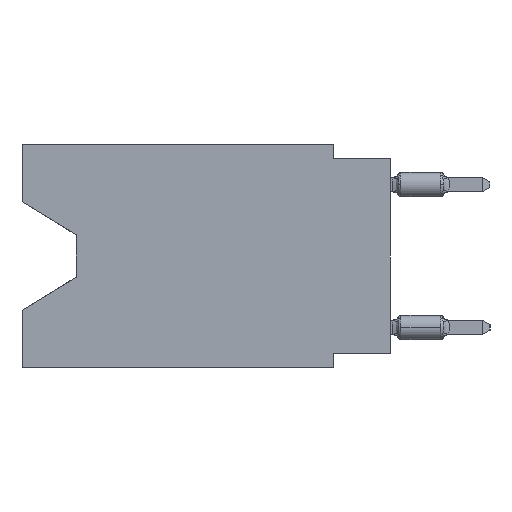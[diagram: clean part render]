
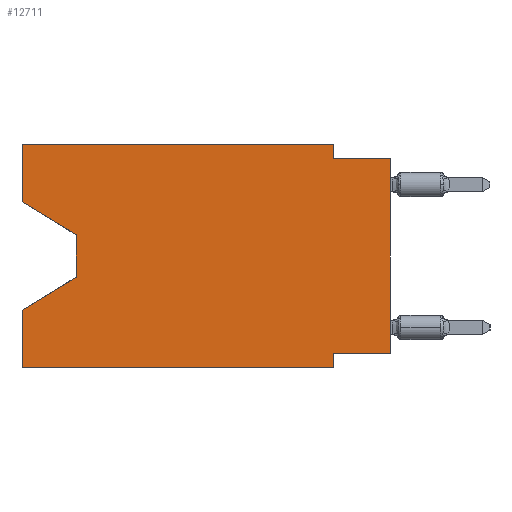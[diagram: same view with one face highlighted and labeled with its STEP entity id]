
A CAD part, left-side view. The second image highlights one B-rep face of the part: STEP entity #12711.
In plain terms, the highlighted planar face has unit normal (-1, 0, 0).
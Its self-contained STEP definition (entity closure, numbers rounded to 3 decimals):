
#188 = CARTESIAN_POINT ( 'NONE',  ( 0., 16.383, 0. ) ) ;
#466 = DIRECTION ( 'NONE',  ( 0., 0., -1. ) ) ;
#687 = EDGE_CURVE ( 'NONE', #22257, #24247, #35026, .T. ) ;
#1067 = CARTESIAN_POINT ( 'NONE',  ( 0., 2.54, -9.271 ) ) ;
#1289 = ORIENTED_EDGE ( 'NONE', *, *, #43319, .F. ) ;
#1474 = CARTESIAN_POINT ( 'NONE',  ( 0., 0., -9.271 ) ) ;
#1740 = CARTESIAN_POINT ( 'NONE',  ( 0., 2.54, 0. ) ) ;
#2173 = CARTESIAN_POINT ( 'NONE',  ( 0., 16.383, -2.546 ) ) ;
#2188 = ORIENTED_EDGE ( 'NONE', *, *, #28853, .F. ) ;
#2395 = DIRECTION ( 'NONE',  ( 0., -0.855, -0.519 ) ) ;
#2905 = DIRECTION ( 'NONE',  ( 0., 0., 1. ) ) ;
#3625 = LINE ( 'NONE', #37755, #48003 ) ;
#3892 = ORIENTED_EDGE ( 'NONE', *, *, #29347, .T. ) ;
#5490 = DIRECTION ( 'NONE',  ( 0., -1., 0. ) ) ;
#5667 = CARTESIAN_POINT ( 'NONE',  ( 0., 16.383, -9.906 ) ) ;
#5978 = AXIS2_PLACEMENT_3D ( 'NONE', #27079, #42142, #466 ) ;
#7020 = FACE_OUTER_BOUND ( 'NONE', #26149, .T. ) ;
#7174 = CARTESIAN_POINT ( 'NONE',  ( 0., 16.383, -2.546 ) ) ;
#7185 = CARTESIAN_POINT ( 'NONE',  ( 0., 16.383, 0. ) ) ;
#8102 = DIRECTION ( 'NONE',  ( 0., 0., -1. ) ) ;
#8670 = DIRECTION ( 'NONE',  ( 0., 0.855, -0.519 ) ) ;
#8674 = DIRECTION ( 'NONE',  ( 0., 0., 1. ) ) ;
#8768 = EDGE_CURVE ( 'NONE', #19900, #25504, #31499, .T. ) ;
#8898 = ORIENTED_EDGE ( 'NONE', *, *, #8768, .T. ) ;
#9522 = CARTESIAN_POINT ( 'NONE',  ( 0., 13.97, -4.013 ) ) ;
#9997 = LINE ( 'NONE', #21544, #36901 ) ;
#10736 = CARTESIAN_POINT ( 'NONE',  ( 0., 16.383, 0. ) ) ;
#11682 = CARTESIAN_POINT ( 'NONE',  ( 0., 0., -9.271 ) ) ;
#11773 = VECTOR ( 'NONE', #8674, 1000. ) ;
#12279 = VECTOR ( 'NONE', #8102, 1000. ) ;
#12711 = ADVANCED_FACE ( 'NONE', ( #7020 ), #19061, .F. ) ;
#13603 = VECTOR ( 'NONE', #16698, 1000. ) ;
#13773 = DIRECTION ( 'NONE',  ( 0., 1., 0. ) ) ;
#15073 = ORIENTED_EDGE ( 'NONE', *, *, #20942, .F. ) ;
#15950 = CARTESIAN_POINT ( 'NONE',  ( 0., 0., 0. ) ) ;
#16143 = EDGE_CURVE ( 'NONE', #34106, #33599, #21721, .T. ) ;
#16698 = DIRECTION ( 'NONE',  ( 0., -1., 0. ) ) ;
#16947 = EDGE_CURVE ( 'NONE', #25840, #47606, #9997, .T. ) ;
#17145 = ORIENTED_EDGE ( 'NONE', *, *, #46094, .F. ) ;
#18259 = VECTOR ( 'NONE', #26549, 1000. ) ;
#18798 = ORIENTED_EDGE ( 'NONE', *, *, #22177, .F. ) ;
#19061 = PLANE ( 'NONE',  #5978 ) ;
#19886 = CARTESIAN_POINT ( 'NONE',  ( 0., 13.97, -5.893 ) ) ;
#19900 = VERTEX_POINT ( 'NONE', #19886 ) ;
#20091 = ORIENTED_EDGE ( 'NONE', *, *, #25852, .F. ) ;
#20136 = ORIENTED_EDGE ( 'NONE', *, *, #687, .T. ) ;
#20232 = LINE ( 'NONE', #5667, #13603 ) ;
#20555 = LINE ( 'NONE', #1474, #39748 ) ;
#20942 = EDGE_CURVE ( 'NONE', #47606, #31670, #43204, .T. ) ;
#21040 = CARTESIAN_POINT ( 'NONE',  ( 0., 0., -0.635 ) ) ;
#21544 = CARTESIAN_POINT ( 'NONE',  ( 0., 16.383, 0. ) ) ;
#21721 = LINE ( 'NONE', #7174, #44094 ) ;
#21752 = VERTEX_POINT ( 'NONE', #41373 ) ;
#22047 = VECTOR ( 'NONE', #36844, 1000. ) ;
#22177 = EDGE_CURVE ( 'NONE', #34106, #25840, #37291, .T. ) ;
#22257 = VERTEX_POINT ( 'NONE', #11682 ) ;
#24247 = VERTEX_POINT ( 'NONE', #48934 ) ;
#25504 = VERTEX_POINT ( 'NONE', #37207 ) ;
#25840 = VERTEX_POINT ( 'NONE', #188 ) ;
#25852 = EDGE_CURVE ( 'NONE', #26384, #25504, #30805, .T. ) ;
#26149 = EDGE_LOOP ( 'NONE', ( #26441, #3892, #8898, #20091, #44015, #2188, #17145, #20136, #1289, #15073, #31025, #18798 ) ) ;
#26181 = CARTESIAN_POINT ( 'NONE',  ( 0., 2.54, -0.635 ) ) ;
#26384 = VERTEX_POINT ( 'NONE', #46529 ) ;
#26441 = ORIENTED_EDGE ( 'NONE', *, *, #16143, .T. ) ;
#26549 = DIRECTION ( 'NONE',  ( 0., 0., 1. ) ) ;
#27079 = CARTESIAN_POINT ( 'NONE',  ( 0., 16.383, 0. ) ) ;
#27192 = VECTOR ( 'NONE', #45726, 1000. ) ;
#28853 = EDGE_CURVE ( 'NONE', #39714, #21752, #3625, .T. ) ;
#29347 = EDGE_CURVE ( 'NONE', #33599, #19900, #30430, .T. ) ;
#29815 = EDGE_CURVE ( 'NONE', #26384, #21752, #20232, .T. ) ;
#30430 = LINE ( 'NONE', #41713, #27192 ) ;
#30806 = VECTOR ( 'NONE', #2905, 1000. ) ;
#30805 = LINE ( 'NONE', #10736, #18259 ) ;
#31025 = ORIENTED_EDGE ( 'NONE', *, *, #16947, .F. ) ;
#31499 = LINE ( 'NONE', #43044, #41835 ) ;
#31670 = VERTEX_POINT ( 'NONE', #26181 ) ;
#31915 = CARTESIAN_POINT ( 'NONE',  ( 0., 2.54, 0. ) ) ;
#33599 = VERTEX_POINT ( 'NONE', #9522 ) ;
#34106 = VERTEX_POINT ( 'NONE', #2173 ) ;
#35026 = LINE ( 'NONE', #15950, #11773 ) ;
#36844 = DIRECTION ( 'NONE',  ( 0., -1., 0. ) ) ;
#36901 = VECTOR ( 'NONE', #5490, 1000. ) ;
#37207 = CARTESIAN_POINT ( 'NONE',  ( 0., 16.383, -7.36 ) ) ;
#37291 = LINE ( 'NONE', #7185, #30806 ) ;
#37755 = CARTESIAN_POINT ( 'NONE',  ( 0., 2.54, -9.906 ) ) ;
#38256 = DIRECTION ( 'NONE',  ( 0., 0., -1. ) ) ;
#39714 = VERTEX_POINT ( 'NONE', #1067 ) ;
#39748 = VECTOR ( 'NONE', #13773, 1000. ) ;
#41373 = CARTESIAN_POINT ( 'NONE',  ( 0., 2.54, -9.906 ) ) ;
#41713 = CARTESIAN_POINT ( 'NONE',  ( 0., 13.97, -4.013 ) ) ;
#41835 = VECTOR ( 'NONE', #8670, 1000. ) ;
#42142 = DIRECTION ( 'NONE',  ( 1., 0., 0. ) ) ;
#43044 = CARTESIAN_POINT ( 'NONE',  ( 0., 13.97, -5.893 ) ) ;
#43204 = LINE ( 'NONE', #31915, #12279 ) ;
#43319 = EDGE_CURVE ( 'NONE', #31670, #24247, #45106, .T. ) ;
#44015 = ORIENTED_EDGE ( 'NONE', *, *, #29815, .T. ) ;
#44094 = VECTOR ( 'NONE', #2395, 1000. ) ;
#45106 = LINE ( 'NONE', #21040, #22047 ) ;
#45726 = DIRECTION ( 'NONE',  ( 0., 0., -1. ) ) ;
#46094 = EDGE_CURVE ( 'NONE', #22257, #39714, #20555, .T. ) ;
#46529 = CARTESIAN_POINT ( 'NONE',  ( 0., 16.383, -9.906 ) ) ;
#47606 = VERTEX_POINT ( 'NONE', #1740 ) ;
#48003 = VECTOR ( 'NONE', #38256, 1000. ) ;
#48934 = CARTESIAN_POINT ( 'NONE',  ( 0., 0., -0.635 ) ) ;
